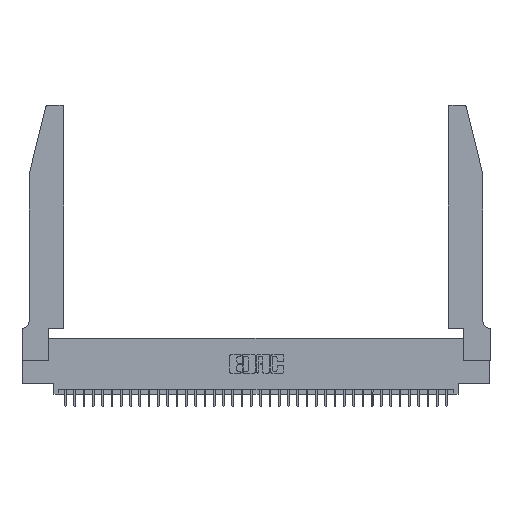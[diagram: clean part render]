
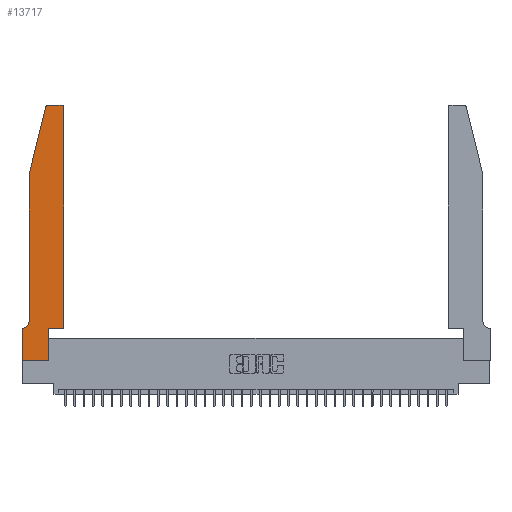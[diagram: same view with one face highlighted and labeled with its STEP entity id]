
A CAD part, top view. The second image highlights one B-rep face of the part: STEP entity #13717.
In plain terms, the highlighted planar face has unit normal (0, 0, 1).
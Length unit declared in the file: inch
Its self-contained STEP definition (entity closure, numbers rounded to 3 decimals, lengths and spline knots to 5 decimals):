
#284 = CARTESIAN_POINT ( 'NONE',  ( 0.0755, 0.42, 0.37 ) ) ;
#482 = CARTESIAN_POINT ( 'NONE',  ( 0.0755, 2., 0.37 ) ) ;
#549 = DIRECTION ( 'NONE',  ( 0., 1., 0. ) ) ;
#737 = CARTESIAN_POINT ( 'NONE',  ( 0.2865, 0.35, 0.37 ) ) ;
#1222 = FACE_OUTER_BOUND ( 'NONE', #6027, .T. ) ;
#1419 = EDGE_CURVE ( 'NONE', #17287, #4540, #25807, .T. ) ;
#2048 = VECTOR ( 'NONE', #25155, 39.37008 ) ;
#2153 = ORIENTED_EDGE ( 'NONE', *, *, #23386, .T. ) ;
#2177 = ORIENTED_EDGE ( 'NONE', *, *, #4527, .T. ) ;
#2353 = LINE ( 'NONE', #28478, #8306 ) ;
#2442 = DIRECTION ( 'NONE',  ( -1., 0., 0. ) ) ;
#2733 = DIRECTION ( 'NONE',  ( 1., 0., 0. ) ) ;
#2759 = ORIENTED_EDGE ( 'NONE', *, *, #33396, .T. ) ;
#2920 = DIRECTION ( 'NONE',  ( 0., 0., 1. ) ) ;
#2989 = EDGE_CURVE ( 'NONE', #7182, #15583, #27101, .T. ) ;
#3290 = VERTEX_POINT ( 'NONE', #11078 ) ;
#4527 = EDGE_CURVE ( 'NONE', #28083, #17287, #6638, .T. ) ;
#4540 = VERTEX_POINT ( 'NONE', #36223 ) ;
#5776 = DIRECTION ( 'NONE',  ( -1., 0., 0. ) ) ;
#6027 = EDGE_LOOP ( 'NONE', ( #2153, #37465, #12675, #2177, #20556, #33043, #33456, #19804, #27172, #2759, #30342, #30141 ) ) ;
#6438 = DIRECTION ( 'NONE',  ( 0., -1., 0. ) ) ;
#6638 = LINE ( 'NONE', #482, #31730 ) ;
#6923 = DIRECTION ( 'NONE',  ( 0., 0., -1. ) ) ;
#7131 = VERTEX_POINT ( 'NONE', #32596 ) ;
#7182 = VERTEX_POINT ( 'NONE', #31864 ) ;
#7445 = LINE ( 'NONE', #15704, #2048 ) ;
#7748 = EDGE_CURVE ( 'NONE', #7131, #7182, #10221, .T. ) ;
#7895 = VERTEX_POINT ( 'NONE', #18651 ) ;
#8301 = DIRECTION ( 'NONE',  ( 0., 0., 1. ) ) ;
#8305 = CARTESIAN_POINT ( 'NONE',  ( 0.284, 2.72, 0.37 ) ) ;
#8306 = VECTOR ( 'NONE', #5776, 39.37008 ) ;
#8389 = LINE ( 'NONE', #28394, #24029 ) ;
#10221 = LINE ( 'NONE', #10597, #32851 ) ;
#10597 = CARTESIAN_POINT ( 'NONE',  ( 0., 0., 0.37 ) ) ;
#10764 = DIRECTION ( 'NONE',  ( 1., 0., 0. ) ) ;
#11078 = CARTESIAN_POINT ( 'NONE',  ( 0., 0.35, 0.37 ) ) ;
#11120 = AXIS2_PLACEMENT_3D ( 'NONE', #22357, #34054, #10764 ) ;
#11227 = LINE ( 'NONE', #28947, #31071 ) ;
#11395 = DIRECTION ( 'NONE',  ( 0., 1., 0. ) ) ;
#12675 = ORIENTED_EDGE ( 'NONE', *, *, #37077, .T. ) ;
#13369 = EDGE_CURVE ( 'NONE', #35289, #32893, #31991, .T. ) ;
#13717 = ADVANCED_FACE ( 'NONE', ( #1222 ), #34624, .T. ) ;
#13765 = EDGE_CURVE ( 'NONE', #32893, #23549, #25811, .T. ) ;
#14126 = AXIS2_PLACEMENT_3D ( 'NONE', #18662, #6923, #21159 ) ;
#15356 = EDGE_CURVE ( 'NONE', #4540, #3290, #8389, .T. ) ;
#15583 = VERTEX_POINT ( 'NONE', #20499 ) ;
#15704 = CARTESIAN_POINT ( 'NONE',  ( 0.4505, 0.35, 0.37 ) ) ;
#16021 = DIRECTION ( 'NONE',  ( 1., 0., 0. ) ) ;
#16345 = LINE ( 'NONE', #25964, #21708 ) ;
#17287 = VERTEX_POINT ( 'NONE', #284 ) ;
#17575 = CARTESIAN_POINT ( 'NONE',  ( 0.4505, 2.72, 0.37 ) ) ;
#18651 = CARTESIAN_POINT ( 'NONE',  ( 0.25487, 2.72718, 0.37 ) ) ;
#18662 = CARTESIAN_POINT ( 'NONE',  ( 0.0055, 0.42, 0.37 ) ) ;
#19071 = CARTESIAN_POINT ( 'NONE',  ( 0.4505, 0.35, 0.37 ) ) ;
#19804 = ORIENTED_EDGE ( 'NONE', *, *, #7748, .T. ) ;
#20499 = CARTESIAN_POINT ( 'NONE',  ( 0.2865, 0.35, 0.37 ) ) ;
#20556 = ORIENTED_EDGE ( 'NONE', *, *, #1419, .T. ) ;
#20810 = CIRCLE ( 'NONE', #26971, 0.03 ) ;
#21159 = DIRECTION ( 'NONE',  ( -1., 0., 0. ) ) ;
#21708 = VECTOR ( 'NONE', #22697, 39.37008 ) ;
#22194 = VECTOR ( 'NONE', #11395, 39.37008 ) ;
#22357 = CARTESIAN_POINT ( 'NONE',  ( 0.4205, 2.72, 0.37 ) ) ;
#22697 = DIRECTION ( 'NONE',  ( 0., -1., 0. ) ) ;
#23386 = EDGE_CURVE ( 'NONE', #23549, #36240, #2353, .T. ) ;
#23549 = VERTEX_POINT ( 'NONE', #26370 ) ;
#24029 = VECTOR ( 'NONE', #2442, 39.37008 ) ;
#25155 = DIRECTION ( 'NONE',  ( 1., 0., 0. ) ) ;
#25268 = CARTESIAN_POINT ( 'NONE',  ( 0.284, 2.75, 0.37 ) ) ;
#25807 = CIRCLE ( 'NONE', #14126, 0.07 ) ;
#25811 = CIRCLE ( 'NONE', #11120, 0.03 ) ;
#25964 = CARTESIAN_POINT ( 'NONE',  ( 0., 0., 0.37 ) ) ;
#26247 = CARTESIAN_POINT ( 'NONE',  ( 0.4505, 0.35, 0.37 ) ) ;
#26370 = CARTESIAN_POINT ( 'NONE',  ( 0.4205, 2.75, 0.37 ) ) ;
#26971 = AXIS2_PLACEMENT_3D ( 'NONE', #8305, #2920, #2733 ) ;
#27101 = LINE ( 'NONE', #737, #27339 ) ;
#27172 = ORIENTED_EDGE ( 'NONE', *, *, #2989, .T. ) ;
#27339 = VECTOR ( 'NONE', #549, 39.37008 ) ;
#28048 = EDGE_CURVE ( 'NONE', #36240, #7895, #20810, .T. ) ;
#28083 = VERTEX_POINT ( 'NONE', #33447 ) ;
#28394 = CARTESIAN_POINT ( 'NONE',  ( 0.0755, 0.35, 0.37 ) ) ;
#28478 = CARTESIAN_POINT ( 'NONE',  ( 0.2605, 2.75, 0.37 ) ) ;
#28947 = CARTESIAN_POINT ( 'NONE',  ( 0.0755, 2., 0.37 ) ) ;
#30141 = ORIENTED_EDGE ( 'NONE', *, *, #13765, .T. ) ;
#30342 = ORIENTED_EDGE ( 'NONE', *, *, #13369, .T. ) ;
#31071 = VECTOR ( 'NONE', #35446, 39.37008 ) ;
#31378 = CARTESIAN_POINT ( 'NONE',  ( 0., 0.35, 0.37 ) ) ;
#31536 = EDGE_CURVE ( 'NONE', #3290, #7131, #16345, .T. ) ;
#31730 = VECTOR ( 'NONE', #6438, 39.37008 ) ;
#31864 = CARTESIAN_POINT ( 'NONE',  ( 0.2865, 0., 0.37 ) ) ;
#31991 = LINE ( 'NONE', #26247, #22194 ) ;
#32024 = AXIS2_PLACEMENT_3D ( 'NONE', #31378, #8301, #34434 ) ;
#32596 = CARTESIAN_POINT ( 'NONE',  ( 0., 0., 0.37 ) ) ;
#32851 = VECTOR ( 'NONE', #16021, 39.37008 ) ;
#32893 = VERTEX_POINT ( 'NONE', #17575 ) ;
#33043 = ORIENTED_EDGE ( 'NONE', *, *, #15356, .T. ) ;
#33396 = EDGE_CURVE ( 'NONE', #15583, #35289, #7445, .T. ) ;
#33447 = CARTESIAN_POINT ( 'NONE',  ( 0.0755, 2., 0.37 ) ) ;
#33456 = ORIENTED_EDGE ( 'NONE', *, *, #31536, .T. ) ;
#34054 = DIRECTION ( 'NONE',  ( 0., 0., 1. ) ) ;
#34434 = DIRECTION ( 'NONE',  ( 1., 0., 0. ) ) ;
#34624 = PLANE ( 'NONE',  #32024 ) ;
#35289 = VERTEX_POINT ( 'NONE', #19071 ) ;
#35446 = DIRECTION ( 'NONE',  ( -0.239, -0.971, 0. ) ) ;
#36223 = CARTESIAN_POINT ( 'NONE',  ( 0.0055, 0.35, 0.37 ) ) ;
#36240 = VERTEX_POINT ( 'NONE', #25268 ) ;
#37077 = EDGE_CURVE ( 'NONE', #7895, #28083, #11227, .T. ) ;
#37465 = ORIENTED_EDGE ( 'NONE', *, *, #28048, .T. ) ;
